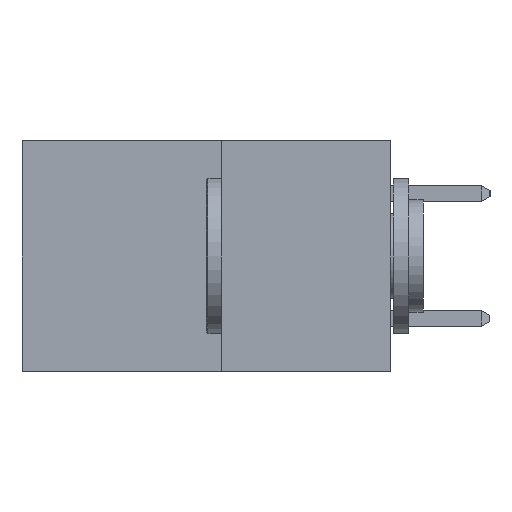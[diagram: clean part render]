
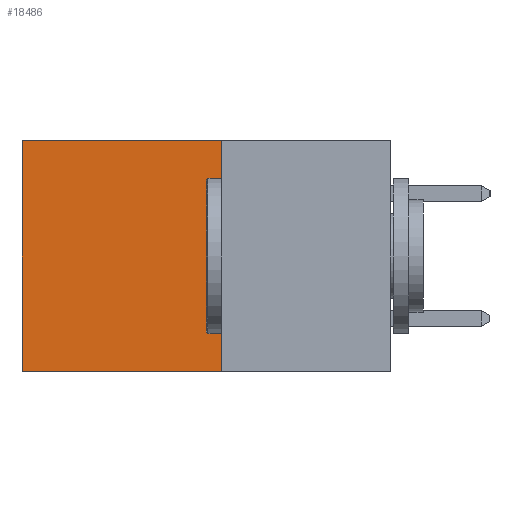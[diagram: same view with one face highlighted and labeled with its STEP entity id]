
A CAD part, left-side view. The second image highlights one B-rep face of the part: STEP entity #18486.
In plain terms, the highlighted planar face has unit normal (-1, 0, 0).
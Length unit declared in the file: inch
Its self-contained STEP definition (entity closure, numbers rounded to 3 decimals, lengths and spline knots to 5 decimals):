
#1098 = CARTESIAN_POINT ( 'NONE',  ( 0.277, 0.59, -0.37 ) ) ;
#1375 = CARTESIAN_POINT ( 'NONE',  ( 0.277, 0.27, 0. ) ) ;
#1685 = VERTEX_POINT ( 'NONE', #7790 ) ;
#1686 = CARTESIAN_POINT ( 'NONE',  ( 0.277, 0.27, -0.37 ) ) ;
#1766 = VERTEX_POINT ( 'NONE', #1098 ) ;
#2731 = LINE ( 'NONE', #16591, #6963 ) ;
#3215 = CARTESIAN_POINT ( 'NONE',  ( 0.277, 0.27, -0.37 ) ) ;
#3374 = DIRECTION ( 'NONE',  ( 0., 0., -1. ) ) ;
#3531 = LINE ( 'NONE', #14994, #16599 ) ;
#4538 = ORIENTED_EDGE ( 'NONE', *, *, #10125, .T. ) ;
#4877 = VECTOR ( 'NONE', #3374, 39.37008 ) ;
#5218 = EDGE_CURVE ( 'NONE', #10749, #8974, #18464, .T. ) ;
#5291 = FACE_OUTER_BOUND ( 'NONE', #17014, .T. ) ;
#5328 = DIRECTION ( 'NONE',  ( 1., 0., 0. ) ) ;
#6963 = VECTOR ( 'NONE', #7784, 39.37008 ) ;
#7784 = DIRECTION ( 'NONE',  ( 0., 1., 0. ) ) ;
#7790 = CARTESIAN_POINT ( 'NONE',  ( 0.277, 0.59, 0. ) ) ;
#8974 = VERTEX_POINT ( 'NONE', #13165 ) ;
#9248 = LINE ( 'NONE', #1375, #18674 ) ;
#10125 = EDGE_CURVE ( 'NONE', #1685, #1766, #3531, .T. ) ;
#10687 = AXIS2_PLACEMENT_3D ( 'NONE', #1686, #5328, #17728 ) ;
#10749 = VERTEX_POINT ( 'NONE', #22205 ) ;
#10938 = ORIENTED_EDGE ( 'NONE', *, *, #16133, .T. ) ;
#11345 = EDGE_CURVE ( 'NONE', #8974, #1766, #2731, .T. ) ;
#11454 = DIRECTION ( 'NONE',  ( 0., 0., -1. ) ) ;
#12104 = DIRECTION ( 'NONE',  ( 0., 1., 0. ) ) ;
#13165 = CARTESIAN_POINT ( 'NONE',  ( 0.277, 0.27, -0.37 ) ) ;
#14994 = CARTESIAN_POINT ( 'NONE',  ( 0.277, 0.59, -0.37 ) ) ;
#15077 = ORIENTED_EDGE ( 'NONE', *, *, #5218, .F. ) ;
#16133 = EDGE_CURVE ( 'NONE', #10749, #1685, #9248, .T. ) ;
#16591 = CARTESIAN_POINT ( 'NONE',  ( 0.277, 0.27, -0.37 ) ) ;
#16599 = VECTOR ( 'NONE', #11454, 39.37008 ) ;
#17014 = EDGE_LOOP ( 'NONE', ( #4538, #18690, #15077, #10938 ) ) ;
#17728 = DIRECTION ( 'NONE',  ( 0., 0., -1. ) ) ;
#18464 = LINE ( 'NONE', #3215, #4877 ) ;
#18486 = ADVANCED_FACE ( 'NONE', ( #5291 ), #19417, .F. ) ;
#18674 = VECTOR ( 'NONE', #12104, 39.37008 ) ;
#18690 = ORIENTED_EDGE ( 'NONE', *, *, #11345, .F. ) ;
#19417 = PLANE ( 'NONE',  #10687 ) ;
#22205 = CARTESIAN_POINT ( 'NONE',  ( 0.277, 0.27, 0. ) ) ;
